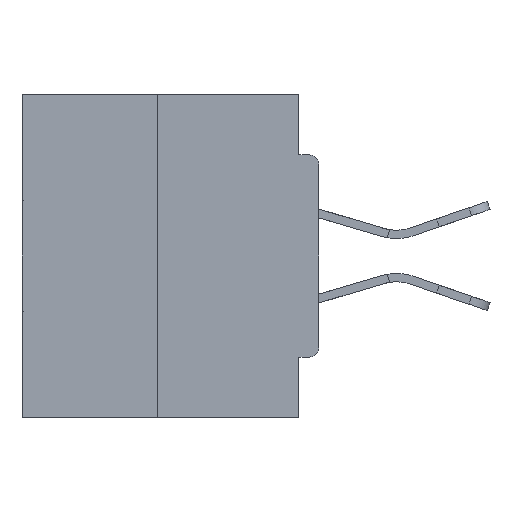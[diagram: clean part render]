
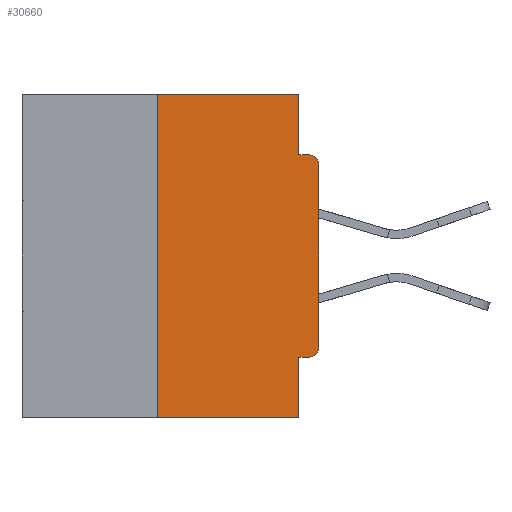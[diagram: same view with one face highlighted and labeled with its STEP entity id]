
A CAD part, left-side view. The second image highlights one B-rep face of the part: STEP entity #30660.
In plain terms, the highlighted planar face has unit normal (-1, 0, 0).
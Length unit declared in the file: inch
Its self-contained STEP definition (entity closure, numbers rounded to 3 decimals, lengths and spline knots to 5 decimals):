
#175 = DIRECTION ( 'NONE',  ( 0., 0., 1. ) ) ;
#328 = LINE ( 'NONE', #15710, #20833 ) ;
#674 = CARTESIAN_POINT ( 'NONE',  ( 0., 0.031, -0.5 ) ) ;
#882 = CARTESIAN_POINT ( 'NONE',  ( 0., 0.46, 0. ) ) ;
#1978 = ORIENTED_EDGE ( 'NONE', *, *, #2266, .F. ) ;
#2266 = EDGE_CURVE ( 'NONE', #33586, #14352, #10388, .T. ) ;
#2498 = VECTOR ( 'NONE', #24433, 39.37008 ) ;
#3438 = CARTESIAN_POINT ( 'NONE',  ( 0., 0.25, 0. ) ) ;
#3476 = ORIENTED_EDGE ( 'NONE', *, *, #38410, .T. ) ;
#3481 = DIRECTION ( 'NONE',  ( 0., -1., 0. ) ) ;
#4073 = AXIS2_PLACEMENT_3D ( 'NONE', #18766, #19164, #34512 ) ;
#5044 = EDGE_CURVE ( 'NONE', #14352, #13582, #18040, .T. ) ;
#5170 = AXIS2_PLACEMENT_3D ( 'NONE', #39059, #20442, #39201 ) ;
#5740 = CARTESIAN_POINT ( 'NONE',  ( 0., 0.031, 0. ) ) ;
#6211 = CIRCLE ( 'NONE', #4073, 0.015 ) ;
#6308 = ORIENTED_EDGE ( 'NONE', *, *, #23607, .T. ) ;
#6394 = LINE ( 'NONE', #26882, #27356 ) ;
#6767 = CARTESIAN_POINT ( 'NONE',  ( 0., 0.46, 0. ) ) ;
#7811 = ORIENTED_EDGE ( 'NONE', *, *, #37310, .T. ) ;
#8084 = CARTESIAN_POINT ( 'NONE',  ( 0., 0., -0.4065 ) ) ;
#10133 = PLANE ( 'NONE',  #40241 ) ;
#10269 = DIRECTION ( 'NONE',  ( 1., 0., 0. ) ) ;
#10324 = ORIENTED_EDGE ( 'NONE', *, *, #35106, .F. ) ;
#10388 = LINE ( 'NONE', #8084, #39127 ) ;
#12472 = CARTESIAN_POINT ( 'NONE',  ( 0., 0.031, -0.5 ) ) ;
#12762 = VERTEX_POINT ( 'NONE', #31345 ) ;
#13005 = VERTEX_POINT ( 'NONE', #25923 ) ;
#13582 = VERTEX_POINT ( 'NONE', #674 ) ;
#14352 = VERTEX_POINT ( 'NONE', #38724 ) ;
#15710 = CARTESIAN_POINT ( 'NONE',  ( 0., 0., 0. ) ) ;
#16186 = EDGE_CURVE ( 'NONE', #32927, #12762, #20718, .T. ) ;
#17079 = EDGE_CURVE ( 'NONE', #38778, #12762, #32297, .T. ) ;
#18040 = LINE ( 'NONE', #12472, #39917 ) ;
#18583 = DIRECTION ( 'NONE',  ( 0., 0., 1. ) ) ;
#18629 = CARTESIAN_POINT ( 'NONE',  ( 0., 0., -0.0935 ) ) ;
#18654 = VERTEX_POINT ( 'NONE', #18836 ) ;
#18766 = CARTESIAN_POINT ( 'NONE',  ( 0., 0.015, -0.3915 ) ) ;
#18836 = CARTESIAN_POINT ( 'NONE',  ( 0., 0.25, -0.5 ) ) ;
#19018 = ORIENTED_EDGE ( 'NONE', *, *, #17079, .F. ) ;
#19044 = LINE ( 'NONE', #6767, #26339 ) ;
#19164 = DIRECTION ( 'NONE',  ( -1., 0., 0. ) ) ;
#19238 = EDGE_CURVE ( 'NONE', #33052, #13005, #19044, .T. ) ;
#19916 = ORIENTED_EDGE ( 'NONE', *, *, #35228, .F. ) ;
#20442 = DIRECTION ( 'NONE',  ( -1., 0., 0. ) ) ;
#20718 = CIRCLE ( 'NONE', #5170, 0.015 ) ;
#20833 = VECTOR ( 'NONE', #18583, 39.37008 ) ;
#20892 = CARTESIAN_POINT ( 'NONE',  ( 0., 0., -0.1085 ) ) ;
#21048 = LINE ( 'NONE', #5740, #2498 ) ;
#21396 = ORIENTED_EDGE ( 'NONE', *, *, #19238, .F. ) ;
#21948 = CARTESIAN_POINT ( 'NONE',  ( 0., 0.25, 0. ) ) ;
#23100 = ORIENTED_EDGE ( 'NONE', *, *, #5044, .F. ) ;
#23607 = EDGE_CURVE ( 'NONE', #18654, #13582, #6394, .T. ) ;
#23745 = DIRECTION ( 'NONE',  ( 0., 1., 0. ) ) ;
#24433 = DIRECTION ( 'NONE',  ( 0., 0., -1. ) ) ;
#24839 = LINE ( 'NONE', #3438, #37504 ) ;
#25277 = DIRECTION ( 'NONE',  ( 0., 0., -1. ) ) ;
#25660 = VERTEX_POINT ( 'NONE', #37548 ) ;
#25923 = CARTESIAN_POINT ( 'NONE',  ( 0., 0.031, 0. ) ) ;
#26339 = VECTOR ( 'NONE', #28562, 39.37008 ) ;
#26343 = DIRECTION ( 'NONE',  ( 0., -1., 0. ) ) ;
#26700 = EDGE_LOOP ( 'NONE', ( #21396, #19916, #6308, #23100, #1978, #3476, #7811, #29905, #19018, #10324 ) ) ;
#26882 = CARTESIAN_POINT ( 'NONE',  ( 0., 0.46, -0.5 ) ) ;
#27356 = VECTOR ( 'NONE', #26343, 39.37008 ) ;
#28562 = DIRECTION ( 'NONE',  ( 0., -1., 0. ) ) ;
#29905 = ORIENTED_EDGE ( 'NONE', *, *, #16186, .T. ) ;
#30324 = VECTOR ( 'NONE', #3481, 39.37008 ) ;
#30660 = ADVANCED_FACE ( 'NONE', ( #39677 ), #10133, .F. ) ;
#31345 = CARTESIAN_POINT ( 'NONE',  ( 0., 0.015, -0.0935 ) ) ;
#32297 = LINE ( 'NONE', #18629, #30324 ) ;
#32682 = CARTESIAN_POINT ( 'NONE',  ( 0., 0.015, -0.4065 ) ) ;
#32927 = VERTEX_POINT ( 'NONE', #20892 ) ;
#33052 = VERTEX_POINT ( 'NONE', #21948 ) ;
#33586 = VERTEX_POINT ( 'NONE', #32682 ) ;
#34512 = DIRECTION ( 'NONE',  ( 0., 0., -1. ) ) ;
#34766 = DIRECTION ( 'NONE',  ( 0., 0., -1. ) ) ;
#35106 = EDGE_CURVE ( 'NONE', #13005, #38778, #21048, .T. ) ;
#35228 = EDGE_CURVE ( 'NONE', #18654, #33052, #24839, .T. ) ;
#36638 = CARTESIAN_POINT ( 'NONE',  ( 0., 0.031, -0.0935 ) ) ;
#37310 = EDGE_CURVE ( 'NONE', #25660, #32927, #328, .T. ) ;
#37504 = VECTOR ( 'NONE', #175, 39.37008 ) ;
#37548 = CARTESIAN_POINT ( 'NONE',  ( 0., 0., -0.3915 ) ) ;
#38410 = EDGE_CURVE ( 'NONE', #33586, #25660, #6211, .T. ) ;
#38724 = CARTESIAN_POINT ( 'NONE',  ( 0., 0.031, -0.4065 ) ) ;
#38778 = VERTEX_POINT ( 'NONE', #36638 ) ;
#39059 = CARTESIAN_POINT ( 'NONE',  ( 0., 0.015, -0.1085 ) ) ;
#39127 = VECTOR ( 'NONE', #23745, 39.37008 ) ;
#39201 = DIRECTION ( 'NONE',  ( 0., 0., -1. ) ) ;
#39677 = FACE_OUTER_BOUND ( 'NONE', #26700, .T. ) ;
#39917 = VECTOR ( 'NONE', #25277, 39.37008 ) ;
#40241 = AXIS2_PLACEMENT_3D ( 'NONE', #882, #10269, #34766 ) ;
